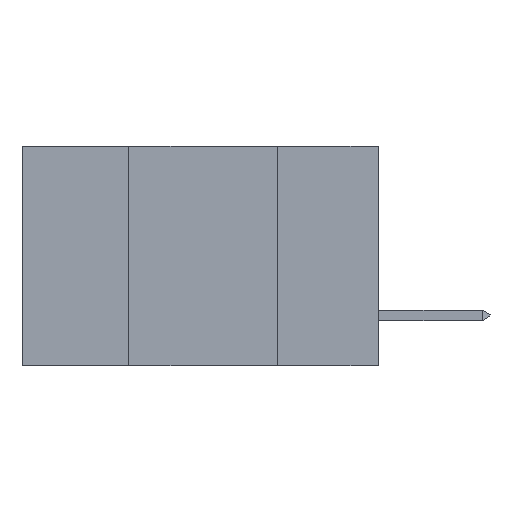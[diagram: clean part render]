
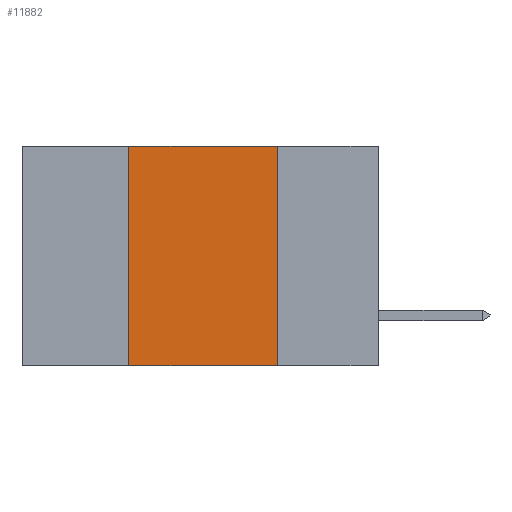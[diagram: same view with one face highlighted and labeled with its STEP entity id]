
A CAD part, left-side view. The second image highlights one B-rep face of the part: STEP entity #11882.
In plain terms, the highlighted planar face has unit normal (-1, 0, 0).
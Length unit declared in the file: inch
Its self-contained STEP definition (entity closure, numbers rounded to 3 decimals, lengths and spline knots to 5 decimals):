
#320 = CARTESIAN_POINT ( 'NONE',  ( 0., 0.42, -0.37 ) ) ;
#351 = ORIENTED_EDGE ( 'NONE', *, *, #3348, .F. ) ;
#1692 = LINE ( 'NONE', #9370, #10045 ) ;
#2020 = AXIS2_PLACEMENT_3D ( 'NONE', #5923, #6902, #8926 ) ;
#2359 = VECTOR ( 'NONE', #4307, 39.37008 ) ;
#2520 = CARTESIAN_POINT ( 'NONE',  ( 0., 0.42, 0. ) ) ;
#2975 = FACE_OUTER_BOUND ( 'NONE', #10857, .T. ) ;
#3348 = EDGE_CURVE ( 'NONE', #9050, #7605, #4783, .T. ) ;
#3352 = ORIENTED_EDGE ( 'NONE', *, *, #5218, .T. ) ;
#3407 = DIRECTION ( 'NONE',  ( 0., 0., -1. ) ) ;
#4307 = DIRECTION ( 'NONE',  ( 0., 0., 1. ) ) ;
#4783 = LINE ( 'NONE', #9528, #9171 ) ;
#4846 = PLANE ( 'NONE',  #2020 ) ;
#5218 = EDGE_CURVE ( 'NONE', #7590, #10131, #6565, .T. ) ;
#5534 = DIRECTION ( 'NONE',  ( 0., -1., 0. ) ) ;
#5671 = ORIENTED_EDGE ( 'NONE', *, *, #8987, .F. ) ;
#5923 = CARTESIAN_POINT ( 'NONE',  ( 0., 0.6, 0. ) ) ;
#6565 = LINE ( 'NONE', #8688, #9696 ) ;
#6902 = DIRECTION ( 'NONE',  ( 1., 0., 0. ) ) ;
#7462 = CARTESIAN_POINT ( 'NONE',  ( 0., 0.42, 0. ) ) ;
#7590 = VERTEX_POINT ( 'NONE', #320 ) ;
#7605 = VERTEX_POINT ( 'NONE', #8279 ) ;
#7708 = LINE ( 'NONE', #7462, #2359 ) ;
#7749 = DIRECTION ( 'NONE',  ( 0., -1., 0. ) ) ;
#8279 = CARTESIAN_POINT ( 'NONE',  ( 0., 0.17, 0. ) ) ;
#8688 = CARTESIAN_POINT ( 'NONE',  ( 0., 0.6, -0.37 ) ) ;
#8926 = DIRECTION ( 'NONE',  ( 0., 0., -1. ) ) ;
#8987 = EDGE_CURVE ( 'NONE', #7590, #9050, #7708, .T. ) ;
#9050 = VERTEX_POINT ( 'NONE', #2520 ) ;
#9171 = VECTOR ( 'NONE', #5534, 39.37008 ) ;
#9264 = CARTESIAN_POINT ( 'NONE',  ( 0., 0.17, -0.37 ) ) ;
#9370 = CARTESIAN_POINT ( 'NONE',  ( 0., 0.17, 0. ) ) ;
#9516 = EDGE_CURVE ( 'NONE', #7605, #10131, #1692, .T. ) ;
#9528 = CARTESIAN_POINT ( 'NONE',  ( 0., 0.6, 0. ) ) ;
#9696 = VECTOR ( 'NONE', #7749, 39.37008 ) ;
#10045 = VECTOR ( 'NONE', #3407, 39.37008 ) ;
#10065 = ORIENTED_EDGE ( 'NONE', *, *, #9516, .F. ) ;
#10131 = VERTEX_POINT ( 'NONE', #9264 ) ;
#10857 = EDGE_LOOP ( 'NONE', ( #10065, #351, #5671, #3352 ) ) ;
#11882 = ADVANCED_FACE ( 'NONE', ( #2975 ), #4846, .F. ) ;
